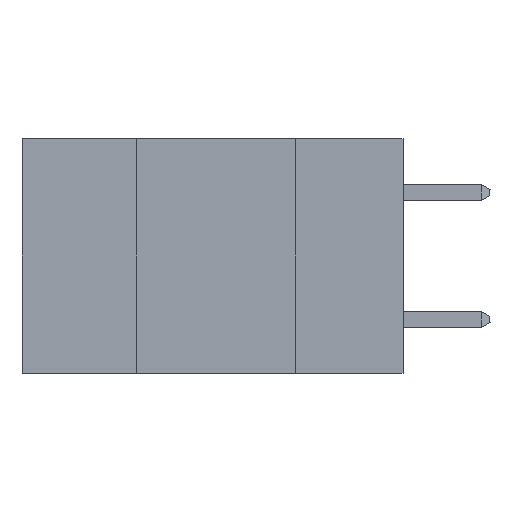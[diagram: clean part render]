
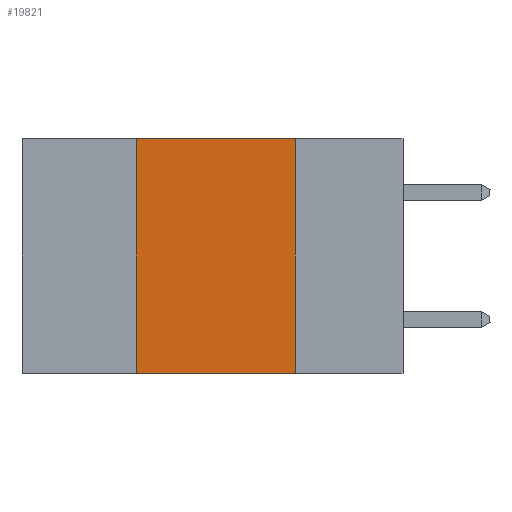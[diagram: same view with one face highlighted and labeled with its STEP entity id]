
A CAD part, left-side view. The second image highlights one B-rep face of the part: STEP entity #19821.
In plain terms, the highlighted planar face has unit normal (-1, 0, 0).
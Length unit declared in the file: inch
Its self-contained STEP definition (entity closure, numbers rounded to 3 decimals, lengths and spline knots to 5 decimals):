
#1276 = DIRECTION ( 'NONE',  ( 1., 0., 0. ) ) ;
#1566 = VERTEX_POINT ( 'NONE', #28705 ) ;
#1837 = DIRECTION ( 'NONE',  ( 0., 0., 1. ) ) ;
#3555 = VECTOR ( 'NONE', #10004, 39.37008 ) ;
#4760 = EDGE_CURVE ( 'NONE', #18925, #39584, #23548, .T. ) ;
#5090 = CARTESIAN_POINT ( 'NONE',  ( 0., 0.42, 0. ) ) ;
#8413 = EDGE_LOOP ( 'NONE', ( #10169, #14906, #20137, #37655 ) ) ;
#9034 = DIRECTION ( 'NONE',  ( 0., -1., 0. ) ) ;
#10004 = DIRECTION ( 'NONE',  ( 0., -1., 0. ) ) ;
#10169 = ORIENTED_EDGE ( 'NONE', *, *, #17831, .F. ) ;
#10801 = CARTESIAN_POINT ( 'NONE',  ( 0., 0.17, 0. ) ) ;
#11056 = DIRECTION ( 'NONE',  ( 0., 0., -1. ) ) ;
#11795 = LINE ( 'NONE', #31632, #3555 ) ;
#13860 = VECTOR ( 'NONE', #26020, 39.37008 ) ;
#14906 = ORIENTED_EDGE ( 'NONE', *, *, #19624, .F. ) ;
#17831 = EDGE_CURVE ( 'NONE', #1566, #39584, #32764, .T. ) ;
#18427 = CARTESIAN_POINT ( 'NONE',  ( 0., 0.6, -0.37 ) ) ;
#18925 = VERTEX_POINT ( 'NONE', #22411 ) ;
#19624 = EDGE_CURVE ( 'NONE', #39681, #1566, #11795, .T. ) ;
#19821 = ADVANCED_FACE ( 'NONE', ( #29167 ), #38436, .F. ) ;
#20137 = ORIENTED_EDGE ( 'NONE', *, *, #37786, .F. ) ;
#21173 = AXIS2_PLACEMENT_3D ( 'NONE', #26261, #1276, #11056 ) ;
#22411 = CARTESIAN_POINT ( 'NONE',  ( 0., 0.42, -0.37 ) ) ;
#23442 = LINE ( 'NONE', #5090, #28757 ) ;
#23548 = LINE ( 'NONE', #18427, #39127 ) ;
#26020 = DIRECTION ( 'NONE',  ( 0., 0., -1. ) ) ;
#26261 = CARTESIAN_POINT ( 'NONE',  ( 0., 0.6, 0. ) ) ;
#28705 = CARTESIAN_POINT ( 'NONE',  ( 0., 0.17, 0. ) ) ;
#28757 = VECTOR ( 'NONE', #1837, 39.37008 ) ;
#29167 = FACE_OUTER_BOUND ( 'NONE', #8413, .T. ) ;
#31632 = CARTESIAN_POINT ( 'NONE',  ( 0., 0.6, 0. ) ) ;
#32764 = LINE ( 'NONE', #10801, #13860 ) ;
#34291 = CARTESIAN_POINT ( 'NONE',  ( 0., 0.17, -0.37 ) ) ;
#37655 = ORIENTED_EDGE ( 'NONE', *, *, #4760, .T. ) ;
#37786 = EDGE_CURVE ( 'NONE', #18925, #39681, #23442, .T. ) ;
#38225 = CARTESIAN_POINT ( 'NONE',  ( 0., 0.42, 0. ) ) ;
#38436 = PLANE ( 'NONE',  #21173 ) ;
#39127 = VECTOR ( 'NONE', #9034, 39.37008 ) ;
#39584 = VERTEX_POINT ( 'NONE', #34291 ) ;
#39681 = VERTEX_POINT ( 'NONE', #38225 ) ;
